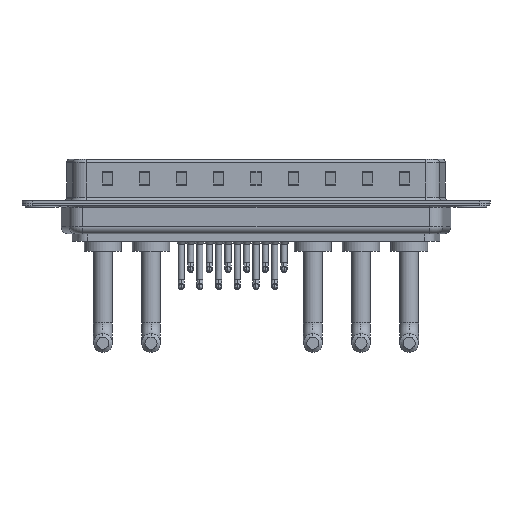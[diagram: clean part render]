
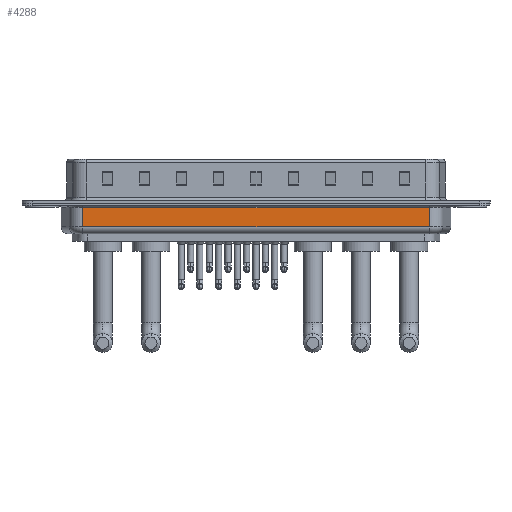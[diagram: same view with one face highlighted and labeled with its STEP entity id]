
A CAD part, front view. The second image highlights one B-rep face of the part: STEP entity #4288.
In plain terms, the highlighted planar face has unit normal (0, -1, 0).
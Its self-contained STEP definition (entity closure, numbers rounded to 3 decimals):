
#973 = AXIS2_PLACEMENT_3D ( 'NONE', #21336, #6258, #19408 ) ;
#1040 = VECTOR ( 'NONE', #17906, 1000. ) ;
#2375 = LINE ( 'NONE', #9726, #9323 ) ;
#2643 = PLANE ( 'NONE',  #973 ) ;
#3179 = ORIENTED_EDGE ( 'NONE', *, *, #6186, .T. ) ;
#4288 = ADVANCED_FACE ( 'NONE', ( #10095 ), #2643, .F. ) ;
#4745 = ORIENTED_EDGE ( 'NONE', *, *, #17854, .F. ) ;
#4991 = LINE ( 'NONE', #12334, #1040 ) ;
#5274 = VERTEX_POINT ( 'NONE', #15845 ) ;
#5302 = VECTOR ( 'NONE', #7657, 1000. ) ;
#5876 = DIRECTION ( 'NONE',  ( 0., 0., 1. ) ) ;
#6186 = EDGE_CURVE ( 'NONE', #9514, #19111, #8632, .T. ) ;
#6258 = DIRECTION ( 'NONE',  ( 0., 1., 0. ) ) ;
#7142 = EDGE_CURVE ( 'NONE', #19111, #5274, #4991, .T. ) ;
#7657 = DIRECTION ( 'NONE',  ( 0., 0., 1. ) ) ;
#8632 = LINE ( 'NONE', #15999, #5302 ) ;
#9323 = VECTOR ( 'NONE', #5876, 1000. ) ;
#9514 = VERTEX_POINT ( 'NONE', #9852 ) ;
#9726 = CARTESIAN_POINT ( 'NONE',  ( 6.031, -5.35, -4.5 ) ) ;
#9852 = CARTESIAN_POINT ( 'NONE',  ( 57.469, -5.35, -3.5 ) ) ;
#10095 = FACE_OUTER_BOUND ( 'NONE', #18126, .T. ) ;
#10295 = ORIENTED_EDGE ( 'NONE', *, *, #7142, .T. ) ;
#11077 = CARTESIAN_POINT ( 'NONE',  ( 6.031, -5.35, -3.5 ) ) ;
#12334 = CARTESIAN_POINT ( 'NONE',  ( 6.031, -5.35, -0.65 ) ) ;
#15203 = VERTEX_POINT ( 'NONE', #17919 ) ;
#15845 = CARTESIAN_POINT ( 'NONE',  ( 6.031, -5.35, -0.65 ) ) ;
#15999 = CARTESIAN_POINT ( 'NONE',  ( 57.469, -5.35, -4.5 ) ) ;
#16754 = ORIENTED_EDGE ( 'NONE', *, *, #22855, .T. ) ;
#17854 = EDGE_CURVE ( 'NONE', #15203, #5274, #2375, .T. ) ;
#17906 = DIRECTION ( 'NONE',  ( -1., 0., 0. ) ) ;
#17919 = CARTESIAN_POINT ( 'NONE',  ( 6.031, -5.35, -3.5 ) ) ;
#18126 = EDGE_LOOP ( 'NONE', ( #4745, #16754, #3179, #10295 ) ) ;
#18824 = CARTESIAN_POINT ( 'NONE',  ( 57.469, -5.35, -0.65 ) ) ;
#19111 = VERTEX_POINT ( 'NONE', #18824 ) ;
#19408 = DIRECTION ( 'NONE',  ( -1., 0., 0. ) ) ;
#20264 = LINE ( 'NONE', #11077, #21789 ) ;
#21336 = CARTESIAN_POINT ( 'NONE',  ( 6.031, -5.35, -4.5 ) ) ;
#21789 = VECTOR ( 'NONE', #23748, 1000. ) ;
#22855 = EDGE_CURVE ( 'NONE', #15203, #9514, #20264, .T. ) ;
#23748 = DIRECTION ( 'NONE',  ( 1., 0., 0. ) ) ;
